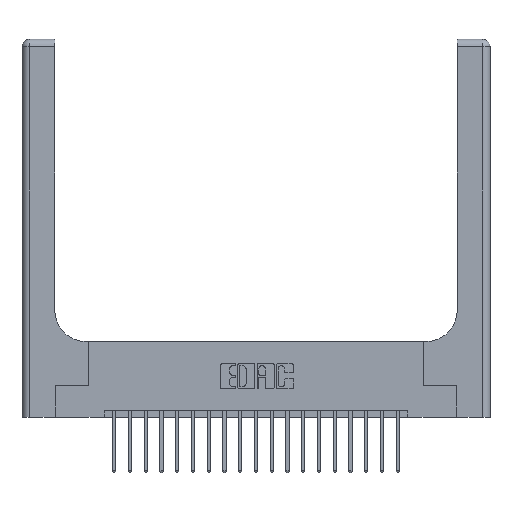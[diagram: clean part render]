
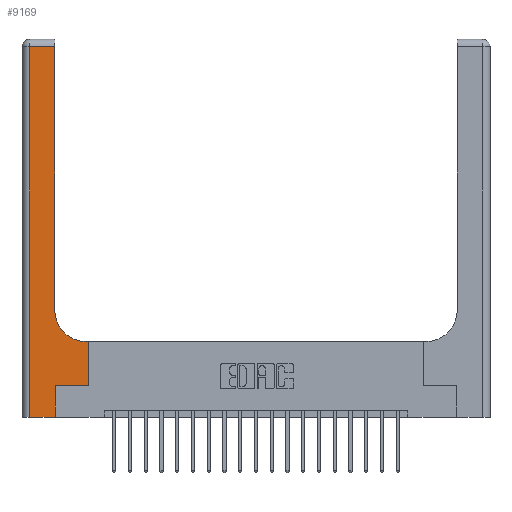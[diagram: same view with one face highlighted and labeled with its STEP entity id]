
A CAD part, top view. The second image highlights one B-rep face of the part: STEP entity #9169.
In plain terms, the highlighted planar face has unit normal (0, 0, 1).
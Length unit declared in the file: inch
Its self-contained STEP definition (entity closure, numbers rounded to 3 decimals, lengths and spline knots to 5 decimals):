
#535 = CARTESIAN_POINT ( 'NONE',  ( 0.265, 0.25, 0.37 ) ) ;
#603 = CARTESIAN_POINT ( 'NONE',  ( 0.528, 0.25, 0.37 ) ) ;
#731 = CIRCLE ( 'NONE', #17822, 0.25 ) ;
#778 = CARTESIAN_POINT ( 'NONE',  ( 0.265, 0.25, 0.37 ) ) ;
#893 = LINE ( 'NONE', #9007, #1913 ) ;
#999 = DIRECTION ( 'NONE',  ( 0., 1., 0. ) ) ;
#1242 = VERTEX_POINT ( 'NONE', #8830 ) ;
#1910 = LINE ( 'NONE', #16465, #17452 ) ;
#1913 = VECTOR ( 'NONE', #20213, 39.37008 ) ;
#3216 = EDGE_CURVE ( 'NONE', #1242, #7712, #16479, .T. ) ;
#4330 = LINE ( 'NONE', #8454, #13891 ) ;
#4433 = CARTESIAN_POINT ( 'NONE',  ( 0.06, 2.94, 0.37 ) ) ;
#4628 = DIRECTION ( 'NONE',  ( 1., 0., 0. ) ) ;
#4660 = EDGE_CURVE ( 'NONE', #7712, #13229, #893, .T. ) ;
#4849 = DIRECTION ( 'NONE',  ( 1., 0., 0. ) ) ;
#5281 = EDGE_CURVE ( 'NONE', #20700, #1242, #4330, .T. ) ;
#5393 = VERTEX_POINT ( 'NONE', #10263 ) ;
#6642 = FACE_OUTER_BOUND ( 'NONE', #12577, .T. ) ;
#7085 = CARTESIAN_POINT ( 'NONE',  ( 0., 3., 0.37 ) ) ;
#7381 = CARTESIAN_POINT ( 'NONE',  ( 0.26, 3., 0.37 ) ) ;
#7391 = ORIENTED_EDGE ( 'NONE', *, *, #17386, .T. ) ;
#7712 = VERTEX_POINT ( 'NONE', #19820 ) ;
#8132 = VERTEX_POINT ( 'NONE', #16169 ) ;
#8234 = EDGE_CURVE ( 'NONE', #10162, #20700, #18985, .T. ) ;
#8454 = CARTESIAN_POINT ( 'NONE',  ( 0.06, 3., 0.37 ) ) ;
#8830 = CARTESIAN_POINT ( 'NONE',  ( 0.06, 0., 0.37 ) ) ;
#9007 = CARTESIAN_POINT ( 'NONE',  ( 0.265, 0., 0.37 ) ) ;
#9147 = ORIENTED_EDGE ( 'NONE', *, *, #3216, .T. ) ;
#9169 = ADVANCED_FACE ( 'NONE', ( #6642 ), #15167, .F. ) ;
#9179 = DIRECTION ( 'NONE',  ( 1., 0., 0. ) ) ;
#9200 = CARTESIAN_POINT ( 'NONE',  ( 0., 2.94, 0.37 ) ) ;
#9284 = AXIS2_PLACEMENT_3D ( 'NONE', #7085, #14054, #20227 ) ;
#9473 = EDGE_CURVE ( 'NONE', #13229, #17692, #19403, .T. ) ;
#10162 = VERTEX_POINT ( 'NONE', #20585 ) ;
#10218 = VECTOR ( 'NONE', #15115, 39.37008 ) ;
#10263 = CARTESIAN_POINT ( 'NONE',  ( 0.51, 0.6, 0.37 ) ) ;
#10692 = VERTEX_POINT ( 'NONE', #11990 ) ;
#11503 = ORIENTED_EDGE ( 'NONE', *, *, #5281, .T. ) ;
#11561 = LINE ( 'NONE', #16626, #15311 ) ;
#11746 = DIRECTION ( 'NONE',  ( 0., -1., 0. ) ) ;
#11990 = CARTESIAN_POINT ( 'NONE',  ( 0.26, 0.85, 0.37 ) ) ;
#12157 = EDGE_CURVE ( 'NONE', #8132, #5393, #11561, .T. ) ;
#12224 = VECTOR ( 'NONE', #9179, 39.37008 ) ;
#12492 = DIRECTION ( 'NONE',  ( -1., 0., 0. ) ) ;
#12577 = EDGE_LOOP ( 'NONE', ( #7391, #17244, #11503, #9147, #13300, #18383, #20249, #20352, #19069 ) ) ;
#13229 = VERTEX_POINT ( 'NONE', #778 ) ;
#13300 = ORIENTED_EDGE ( 'NONE', *, *, #4660, .T. ) ;
#13688 = VECTOR ( 'NONE', #12492, 39.37008 ) ;
#13891 = VECTOR ( 'NONE', #11746, 39.37008 ) ;
#14054 = DIRECTION ( 'NONE',  ( 0., 0., -1. ) ) ;
#14248 = CARTESIAN_POINT ( 'NONE',  ( 0.51, 0.85, 0.37 ) ) ;
#15115 = DIRECTION ( 'NONE',  ( 0., 1., 0. ) ) ;
#15167 = PLANE ( 'NONE',  #9284 ) ;
#15311 = VECTOR ( 'NONE', #18238, 39.37008 ) ;
#15721 = LINE ( 'NONE', #7381, #10218 ) ;
#16169 = CARTESIAN_POINT ( 'NONE',  ( 0.528, 0.6, 0.37 ) ) ;
#16465 = CARTESIAN_POINT ( 'NONE',  ( 0.528, 0.25, 0.37 ) ) ;
#16479 = LINE ( 'NONE', #17102, #12224 ) ;
#16626 = CARTESIAN_POINT ( 'NONE',  ( 0.26, 0.6, 0.37 ) ) ;
#16883 = EDGE_CURVE ( 'NONE', #5393, #10692, #731, .T. ) ;
#17102 = CARTESIAN_POINT ( 'NONE',  ( 0., 0., 0.37 ) ) ;
#17244 = ORIENTED_EDGE ( 'NONE', *, *, #8234, .T. ) ;
#17386 = EDGE_CURVE ( 'NONE', #10692, #10162, #15721, .T. ) ;
#17452 = VECTOR ( 'NONE', #999, 39.37008 ) ;
#17675 = VECTOR ( 'NONE', #4849, 39.37008 ) ;
#17692 = VERTEX_POINT ( 'NONE', #603 ) ;
#17822 = AXIS2_PLACEMENT_3D ( 'NONE', #14248, #19174, #4628 ) ;
#18238 = DIRECTION ( 'NONE',  ( -1., 0., 0. ) ) ;
#18383 = ORIENTED_EDGE ( 'NONE', *, *, #9473, .T. ) ;
#18985 = LINE ( 'NONE', #9200, #13688 ) ;
#19069 = ORIENTED_EDGE ( 'NONE', *, *, #16883, .T. ) ;
#19084 = EDGE_CURVE ( 'NONE', #17692, #8132, #1910, .T. ) ;
#19174 = DIRECTION ( 'NONE',  ( 0., 0., -1. ) ) ;
#19403 = LINE ( 'NONE', #535, #17675 ) ;
#19820 = CARTESIAN_POINT ( 'NONE',  ( 0.265, 0., 0.37 ) ) ;
#20213 = DIRECTION ( 'NONE',  ( 0., 1., 0. ) ) ;
#20227 = DIRECTION ( 'NONE',  ( -1., 0., 0. ) ) ;
#20249 = ORIENTED_EDGE ( 'NONE', *, *, #19084, .T. ) ;
#20352 = ORIENTED_EDGE ( 'NONE', *, *, #12157, .T. ) ;
#20585 = CARTESIAN_POINT ( 'NONE',  ( 0.26, 2.94, 0.37 ) ) ;
#20700 = VERTEX_POINT ( 'NONE', #4433 ) ;
